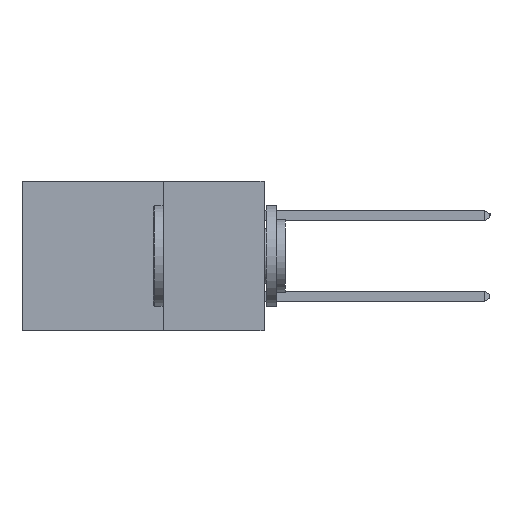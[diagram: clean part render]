
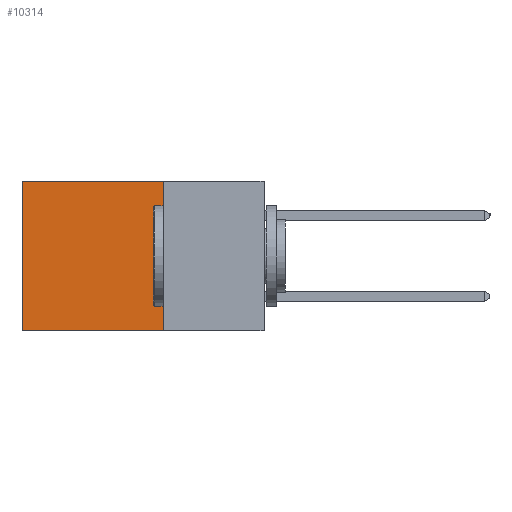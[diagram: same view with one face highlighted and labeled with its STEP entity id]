
A CAD part, left-side view. The second image highlights one B-rep face of the part: STEP entity #10314.
In plain terms, the highlighted planar face has unit normal (-1, 0, 0).
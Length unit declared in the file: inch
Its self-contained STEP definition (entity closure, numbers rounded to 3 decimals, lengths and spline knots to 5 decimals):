
#76 = DIRECTION ( 'NONE',  ( 0., 0., -1. ) ) ;
#463 = VERTEX_POINT ( 'NONE', #13090 ) ;
#1492 = CARTESIAN_POINT ( 'NONE',  ( 0.2615, 0.6, 0. ) ) ;
#1541 = LINE ( 'NONE', #11638, #5818 ) ;
#2376 = LINE ( 'NONE', #7831, #12256 ) ;
#3093 = VERTEX_POINT ( 'NONE', #14106 ) ;
#4158 = DIRECTION ( 'NONE',  ( 0., 1., 0. ) ) ;
#4460 = CARTESIAN_POINT ( 'NONE',  ( 0.2615, 0.25, 0. ) ) ;
#4956 = EDGE_CURVE ( 'NONE', #3093, #10649, #2376, .T. ) ;
#5389 = EDGE_CURVE ( 'NONE', #463, #19014, #17767, .T. ) ;
#5522 = EDGE_CURVE ( 'NONE', #463, #3093, #1541, .T. ) ;
#5818 = VECTOR ( 'NONE', #8364, 39.37008 ) ;
#5961 = CARTESIAN_POINT ( 'NONE',  ( 0.2615, 0.6, -0.37 ) ) ;
#7664 = DIRECTION ( 'NONE',  ( 1., 0., 0. ) ) ;
#7831 = CARTESIAN_POINT ( 'NONE',  ( 0.2615, 0.25, -0.37 ) ) ;
#8364 = DIRECTION ( 'NONE',  ( 0., 0., -1. ) ) ;
#8824 = EDGE_CURVE ( 'NONE', #19014, #10649, #15498, .T. ) ;
#9390 = DIRECTION ( 'NONE',  ( 0., 1., 0. ) ) ;
#9470 = FACE_OUTER_BOUND ( 'NONE', #10670, .T. ) ;
#10120 = ORIENTED_EDGE ( 'NONE', *, *, #5522, .F. ) ;
#10314 = ADVANCED_FACE ( 'NONE', ( #9470 ), #16380, .F. ) ;
#10649 = VERTEX_POINT ( 'NONE', #5961 ) ;
#10670 = EDGE_LOOP ( 'NONE', ( #21612, #14964, #10120, #21384 ) ) ;
#11617 = VECTOR ( 'NONE', #76, 39.37008 ) ;
#11638 = CARTESIAN_POINT ( 'NONE',  ( 0.2615, 0.25, -0.37 ) ) ;
#12256 = VECTOR ( 'NONE', #4158, 39.37008 ) ;
#12819 = DIRECTION ( 'NONE',  ( 0., 0., -1. ) ) ;
#13090 = CARTESIAN_POINT ( 'NONE',  ( 0.2615, 0.25, 0. ) ) ;
#14106 = CARTESIAN_POINT ( 'NONE',  ( 0.2615, 0.25, -0.37 ) ) ;
#14374 = AXIS2_PLACEMENT_3D ( 'NONE', #17829, #7664, #12819 ) ;
#14964 = ORIENTED_EDGE ( 'NONE', *, *, #4956, .F. ) ;
#15498 = LINE ( 'NONE', #17494, #11617 ) ;
#16380 = PLANE ( 'NONE',  #14374 ) ;
#16542 = VECTOR ( 'NONE', #9390, 39.37008 ) ;
#17494 = CARTESIAN_POINT ( 'NONE',  ( 0.2615, 0.6, -0.37 ) ) ;
#17767 = LINE ( 'NONE', #4460, #16542 ) ;
#17829 = CARTESIAN_POINT ( 'NONE',  ( 0.2615, 0.25, -0.37 ) ) ;
#19014 = VERTEX_POINT ( 'NONE', #1492 ) ;
#21384 = ORIENTED_EDGE ( 'NONE', *, *, #5389, .T. ) ;
#21612 = ORIENTED_EDGE ( 'NONE', *, *, #8824, .T. ) ;
